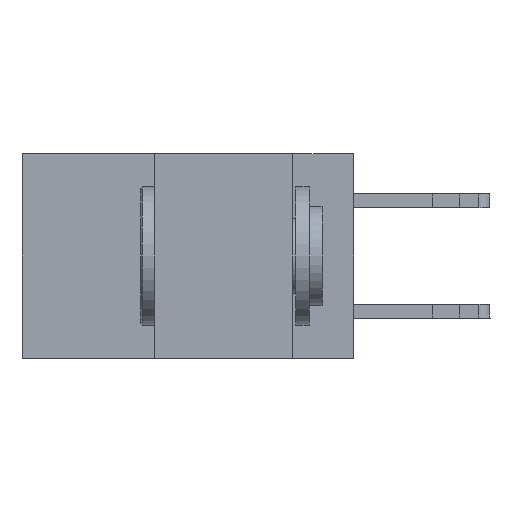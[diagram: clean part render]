
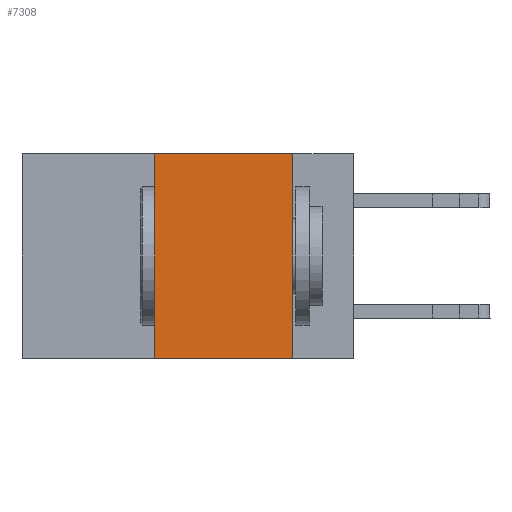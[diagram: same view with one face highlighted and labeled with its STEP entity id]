
A CAD part, left-side view. The second image highlights one B-rep face of the part: STEP entity #7308.
In plain terms, the highlighted planar face has unit normal (-1, 0, 0).
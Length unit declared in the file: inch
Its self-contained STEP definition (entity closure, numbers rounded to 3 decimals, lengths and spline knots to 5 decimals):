
#2037 = VERTEX_POINT ( 'NONE', #7601 ) ;
#2212 = VERTEX_POINT ( 'NONE', #11437 ) ;
#3286 = CARTESIAN_POINT ( 'NONE',  ( 0., 0.11, -0.37 ) ) ;
#3700 = CARTESIAN_POINT ( 'NONE',  ( 0., 0.36, 0. ) ) ;
#3784 = VECTOR ( 'NONE', #12229, 39.37008 ) ;
#4516 = CARTESIAN_POINT ( 'NONE',  ( 0., 0.6, -0.37 ) ) ;
#4792 = CARTESIAN_POINT ( 'NONE',  ( 0., 0.6, 0. ) ) ;
#7308 = ADVANCED_FACE ( 'NONE', ( #33547 ), #9748, .F. ) ;
#7558 = VERTEX_POINT ( 'NONE', #3286 ) ;
#7594 = VECTOR ( 'NONE', #9395, 39.37008 ) ;
#7601 = CARTESIAN_POINT ( 'NONE',  ( 0., 0.11, 0. ) ) ;
#7819 = LINE ( 'NONE', #4516, #3784 ) ;
#9395 = DIRECTION ( 'NONE',  ( 0., -1., 0. ) ) ;
#9748 = PLANE ( 'NONE',  #20604 ) ;
#11437 = CARTESIAN_POINT ( 'NONE',  ( 0., 0.36, -0.37 ) ) ;
#12004 = VERTEX_POINT ( 'NONE', #29438 ) ;
#12178 = DIRECTION ( 'NONE',  ( 0., 0., -1. ) ) ;
#12229 = DIRECTION ( 'NONE',  ( 0., -1., 0. ) ) ;
#12794 = EDGE_CURVE ( 'NONE', #12004, #2037, #14545, .T. ) ;
#12974 = ORIENTED_EDGE ( 'NONE', *, *, #20884, .F. ) ;
#13411 = EDGE_LOOP ( 'NONE', ( #15367, #28643, #12974, #29661 ) ) ;
#14545 = LINE ( 'NONE', #25282, #7594 ) ;
#14677 = DIRECTION ( 'NONE',  ( 1., 0., 0. ) ) ;
#15367 = ORIENTED_EDGE ( 'NONE', *, *, #24803, .F. ) ;
#15536 = EDGE_CURVE ( 'NONE', #2212, #7558, #7819, .T. ) ;
#18527 = VECTOR ( 'NONE', #21918, 39.37008 ) ;
#18707 = CARTESIAN_POINT ( 'NONE',  ( 0., 0.11, 0. ) ) ;
#20604 = AXIS2_PLACEMENT_3D ( 'NONE', #4792, #14677, #12178 ) ;
#20884 = EDGE_CURVE ( 'NONE', #2212, #12004, #26668, .T. ) ;
#21317 = VECTOR ( 'NONE', #22252, 39.37008 ) ;
#21918 = DIRECTION ( 'NONE',  ( 0., 0., 1. ) ) ;
#22252 = DIRECTION ( 'NONE',  ( 0., 0., -1. ) ) ;
#24803 = EDGE_CURVE ( 'NONE', #2037, #7558, #31942, .T. ) ;
#25282 = CARTESIAN_POINT ( 'NONE',  ( 0., 0.6, 0. ) ) ;
#26668 = LINE ( 'NONE', #3700, #18527 ) ;
#28643 = ORIENTED_EDGE ( 'NONE', *, *, #12794, .F. ) ;
#29438 = CARTESIAN_POINT ( 'NONE',  ( 0., 0.36, 0. ) ) ;
#29661 = ORIENTED_EDGE ( 'NONE', *, *, #15536, .T. ) ;
#31942 = LINE ( 'NONE', #18707, #21317 ) ;
#33547 = FACE_OUTER_BOUND ( 'NONE', #13411, .T. ) ;
